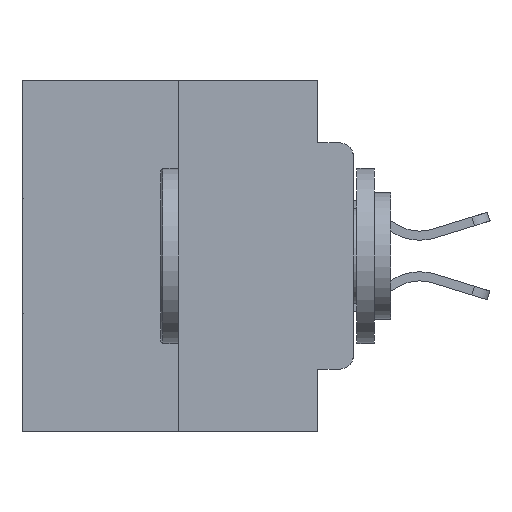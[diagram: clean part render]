
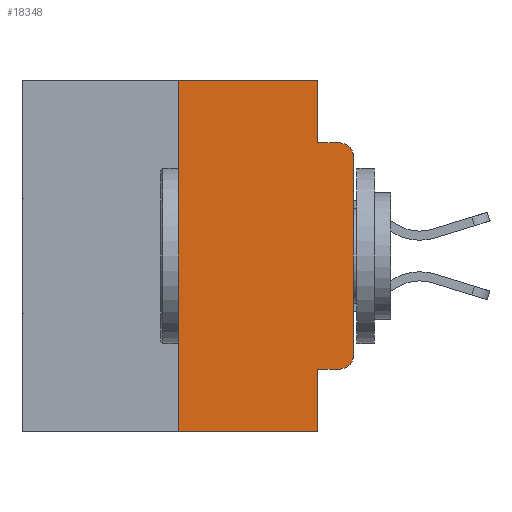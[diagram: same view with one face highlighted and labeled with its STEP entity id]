
A CAD part, left-side view. The second image highlights one B-rep face of the part: STEP entity #18348.
In plain terms, the highlighted planar face has unit normal (-1, 0, 0).
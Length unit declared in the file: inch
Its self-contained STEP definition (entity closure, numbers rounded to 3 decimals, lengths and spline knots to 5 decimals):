
#617 = VERTEX_POINT ( 'NONE', #3137 ) ;
#651 = EDGE_CURVE ( 'NONE', #21402, #2331, #11072, .T. ) ;
#922 = DIRECTION ( 'NONE',  ( 0., -1., 0. ) ) ;
#2331 = VERTEX_POINT ( 'NONE', #17932 ) ;
#2951 = LINE ( 'NONE', #12445, #9398 ) ;
#3127 = CARTESIAN_POINT ( 'NONE',  ( 0., 0.25, 0. ) ) ;
#3137 = CARTESIAN_POINT ( 'NONE',  ( 0., 0.25, 0. ) ) ;
#3167 = CARTESIAN_POINT ( 'NONE',  ( 0., 0.051, 0. ) ) ;
#3239 = CARTESIAN_POINT ( 'NONE',  ( 0., 0.051, -0.4115 ) ) ;
#4271 = EDGE_CURVE ( 'NONE', #9394, #21801, #11598, .T. ) ;
#4543 = FACE_OUTER_BOUND ( 'NONE', #13128, .T. ) ;
#4656 = DIRECTION ( 'NONE',  ( 1., 0., 0. ) ) ;
#5257 = VECTOR ( 'NONE', #20369, 39.37008 ) ;
#5522 = EDGE_CURVE ( 'NONE', #20727, #27812, #25594, .T. ) ;
#6481 = EDGE_CURVE ( 'NONE', #27812, #21402, #17073, .T. ) ;
#6610 = ORIENTED_EDGE ( 'NONE', *, *, #4271, .F. ) ;
#7137 = CARTESIAN_POINT ( 'NONE',  ( 0., 0.02, -0.4115 ) ) ;
#7157 = DIRECTION ( 'NONE',  ( -1., 0., 0. ) ) ;
#7846 = VECTOR ( 'NONE', #922, 39.37008 ) ;
#7929 = ORIENTED_EDGE ( 'NONE', *, *, #5522, .T. ) ;
#8104 = DIRECTION ( 'NONE',  ( 0., -1., 0. ) ) ;
#8113 = EDGE_CURVE ( 'NONE', #617, #9682, #26105, .T. ) ;
#8496 = CARTESIAN_POINT ( 'NONE',  ( 0., 0., 0. ) ) ;
#8513 = LINE ( 'NONE', #20510, #7846 ) ;
#8633 = VECTOR ( 'NONE', #14031, 39.37008 ) ;
#8845 = VECTOR ( 'NONE', #8104, 39.37008 ) ;
#8924 = ORIENTED_EDGE ( 'NONE', *, *, #651, .T. ) ;
#9394 = VERTEX_POINT ( 'NONE', #23274 ) ;
#9398 = VECTOR ( 'NONE', #25447, 39.37008 ) ;
#9682 = VERTEX_POINT ( 'NONE', #3167 ) ;
#10232 = ORIENTED_EDGE ( 'NONE', *, *, #8113, .F. ) ;
#10297 = EDGE_CURVE ( 'NONE', #15957, #21801, #20243, .T. ) ;
#11072 = CIRCLE ( 'NONE', #12826, 0.02 ) ;
#11513 = CARTESIAN_POINT ( 'NONE',  ( 0., 0., -0.1085 ) ) ;
#11598 = LINE ( 'NONE', #22553, #5257 ) ;
#11821 = DIRECTION ( 'NONE',  ( 0., -1., 0. ) ) ;
#12146 = EDGE_CURVE ( 'NONE', #9394, #20727, #14321, .T. ) ;
#12445 = CARTESIAN_POINT ( 'NONE',  ( 0., 0.051, 0. ) ) ;
#12826 = AXIS2_PLACEMENT_3D ( 'NONE', #18576, #13738, #13705 ) ;
#13128 = EDGE_LOOP ( 'NONE', ( #24836, #8924, #20473, #26844, #10232, #21841, #16703, #6610, #18085, #7929 ) ) ;
#13705 = DIRECTION ( 'NONE',  ( 0., 0., -1. ) ) ;
#13738 = DIRECTION ( 'NONE',  ( -1., 0., 0. ) ) ;
#13737 = CARTESIAN_POINT ( 'NONE',  ( 0., 0.473, -0.5 ) ) ;
#13835 = DIRECTION ( 'NONE',  ( 0., -1., 0. ) ) ;
#14031 = DIRECTION ( 'NONE',  ( 0., 0., 1. ) ) ;
#14321 = LINE ( 'NONE', #3239, #25830 ) ;
#14388 = LINE ( 'NONE', #3127, #8633 ) ;
#15957 = VERTEX_POINT ( 'NONE', #20079 ) ;
#16703 = ORIENTED_EDGE ( 'NONE', *, *, #10297, .T. ) ;
#16941 = VERTEX_POINT ( 'NONE', #23719 ) ;
#17073 = LINE ( 'NONE', #8496, #27862 ) ;
#17294 = EDGE_CURVE ( 'NONE', #15957, #617, #14388, .T. ) ;
#17582 = CARTESIAN_POINT ( 'NONE',  ( 0., 0.473, 0. ) ) ;
#17932 = CARTESIAN_POINT ( 'NONE',  ( 0., 0.02, -0.0885 ) ) ;
#18085 = ORIENTED_EDGE ( 'NONE', *, *, #12146, .T. ) ;
#18348 = ADVANCED_FACE ( 'NONE', ( #4543 ), #21882, .F. ) ;
#18576 = CARTESIAN_POINT ( 'NONE',  ( 0., 0.02, -0.1085 ) ) ;
#19558 = VECTOR ( 'NONE', #13835, 39.37008 ) ;
#19760 = DIRECTION ( 'NONE',  ( 0., 0., -1. ) ) ;
#20079 = CARTESIAN_POINT ( 'NONE',  ( 0., 0.25, -0.5 ) ) ;
#20103 = CARTESIAN_POINT ( 'NONE',  ( 0., 0.02, -0.3915 ) ) ;
#20243 = LINE ( 'NONE', #13737, #19558 ) ;
#20369 = DIRECTION ( 'NONE',  ( 0., 0., -1. ) ) ;
#20473 = ORIENTED_EDGE ( 'NONE', *, *, #25453, .F. ) ;
#20510 = CARTESIAN_POINT ( 'NONE',  ( 0., 0.051, -0.0885 ) ) ;
#20727 = VERTEX_POINT ( 'NONE', #7137 ) ;
#20999 = CARTESIAN_POINT ( 'NONE',  ( 0., 0.473, 0. ) ) ;
#21402 = VERTEX_POINT ( 'NONE', #11513 ) ;
#21690 = EDGE_CURVE ( 'NONE', #9682, #16941, #2951, .T. ) ;
#21801 = VERTEX_POINT ( 'NONE', #25818 ) ;
#21841 = ORIENTED_EDGE ( 'NONE', *, *, #17294, .F. ) ;
#21882 = PLANE ( 'NONE',  #22881 ) ;
#22292 = DIRECTION ( 'NONE',  ( 0., 0., -1. ) ) ;
#22553 = CARTESIAN_POINT ( 'NONE',  ( 0., 0.051, 0. ) ) ;
#22881 = AXIS2_PLACEMENT_3D ( 'NONE', #17582, #4656, #19760 ) ;
#23274 = CARTESIAN_POINT ( 'NONE',  ( 0., 0.051, -0.4115 ) ) ;
#23719 = CARTESIAN_POINT ( 'NONE',  ( 0., 0.051, -0.0885 ) ) ;
#24796 = AXIS2_PLACEMENT_3D ( 'NONE', #20103, #7157, #22292 ) ;
#24836 = ORIENTED_EDGE ( 'NONE', *, *, #6481, .T. ) ;
#25447 = DIRECTION ( 'NONE',  ( 0., 0., -1. ) ) ;
#25453 = EDGE_CURVE ( 'NONE', #16941, #2331, #8513, .T. ) ;
#25594 = CIRCLE ( 'NONE', #24796, 0.02 ) ;
#25808 = DIRECTION ( 'NONE',  ( 0., 0., 1. ) ) ;
#25818 = CARTESIAN_POINT ( 'NONE',  ( 0., 0.051, -0.5 ) ) ;
#25830 = VECTOR ( 'NONE', #11821, 39.37008 ) ;
#26105 = LINE ( 'NONE', #20999, #8845 ) ;
#26844 = ORIENTED_EDGE ( 'NONE', *, *, #21690, .F. ) ;
#27812 = VERTEX_POINT ( 'NONE', #28023 ) ;
#27862 = VECTOR ( 'NONE', #25808, 39.37008 ) ;
#28023 = CARTESIAN_POINT ( 'NONE',  ( 0., 0., -0.3915 ) ) ;
